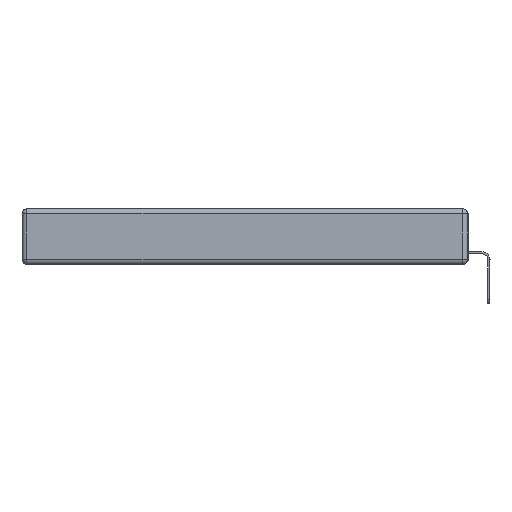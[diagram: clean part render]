
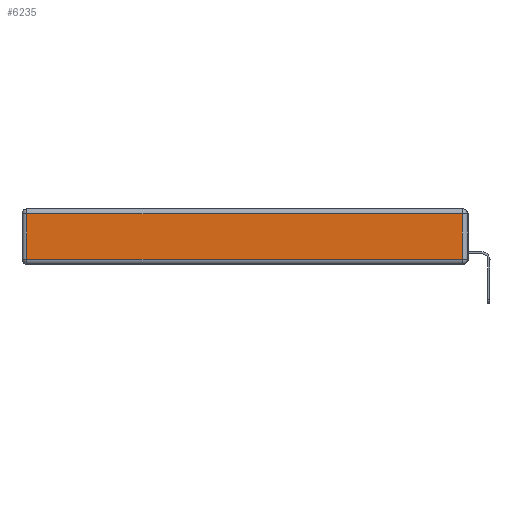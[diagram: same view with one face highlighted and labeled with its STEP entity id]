
A CAD part, left-side view. The second image highlights one B-rep face of the part: STEP entity #6235.
In plain terms, the highlighted planar face has unit normal (-1, 0, 0).
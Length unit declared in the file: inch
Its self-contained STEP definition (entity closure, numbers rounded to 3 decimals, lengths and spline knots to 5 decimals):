
#441 = VECTOR ( 'NONE', #6991, 39.37008 ) ;
#1010 = AXIS2_PLACEMENT_3D ( 'NONE', #11171, #18867, #4744 ) ;
#1175 = FACE_OUTER_BOUND ( 'NONE', #8351, .T. ) ;
#1497 = VERTEX_POINT ( 'NONE', #19045 ) ;
#2666 = DIRECTION ( 'NONE',  ( 0., 0., -1. ) ) ;
#3133 = PLANE ( 'NONE',  #1010 ) ;
#4744 = DIRECTION ( 'NONE',  ( 0., 0., 1. ) ) ;
#5051 = VERTEX_POINT ( 'NONE', #17936 ) ;
#5060 = DIRECTION ( 'NONE',  ( 0., -1., 0. ) ) ;
#5357 = VECTOR ( 'NONE', #15105, 39.37008 ) ;
#5950 = CARTESIAN_POINT ( 'NONE',  ( 0., 2.72, -0.343 ) ) ;
#6235 = ADVANCED_FACE ( 'NONE', ( #1175 ), #3133, .T. ) ;
#6850 = EDGE_CURVE ( 'NONE', #5051, #15081, #16996, .T. ) ;
#6991 = DIRECTION ( 'NONE',  ( 0., 1., 0. ) ) ;
#8351 = EDGE_LOOP ( 'NONE', ( #13451, #8985, #16071, #19048 ) ) ;
#8985 = ORIENTED_EDGE ( 'NONE', *, *, #14869, .T. ) ;
#9962 = CARTESIAN_POINT ( 'NONE',  ( 0., 0.03, -0.03 ) ) ;
#10118 = LINE ( 'NONE', #14499, #5357 ) ;
#11171 = CARTESIAN_POINT ( 'NONE',  ( 0., 0., -0.343 ) ) ;
#12947 = EDGE_CURVE ( 'NONE', #17472, #1497, #17283, .T. ) ;
#13451 = ORIENTED_EDGE ( 'NONE', *, *, #6850, .T. ) ;
#14499 = CARTESIAN_POINT ( 'NONE',  ( 0., 0.03, -0.343 ) ) ;
#14869 = EDGE_CURVE ( 'NONE', #15081, #17472, #10118, .T. ) ;
#15017 = VECTOR ( 'NONE', #5060, 39.37008 ) ;
#15081 = VERTEX_POINT ( 'NONE', #15450 ) ;
#15105 = DIRECTION ( 'NONE',  ( 0., 0., 1. ) ) ;
#15450 = CARTESIAN_POINT ( 'NONE',  ( 0., 0.03, -0.313 ) ) ;
#15905 = VECTOR ( 'NONE', #2666, 39.37008 ) ;
#16071 = ORIENTED_EDGE ( 'NONE', *, *, #12947, .T. ) ;
#16996 = LINE ( 'NONE', #17722, #15017 ) ;
#17283 = LINE ( 'NONE', #19730, #441 ) ;
#17472 = VERTEX_POINT ( 'NONE', #9962 ) ;
#17710 = EDGE_CURVE ( 'NONE', #1497, #5051, #18639, .T. ) ;
#17722 = CARTESIAN_POINT ( 'NONE',  ( 0., 0., -0.313 ) ) ;
#17936 = CARTESIAN_POINT ( 'NONE',  ( 0., 2.72, -0.313 ) ) ;
#18639 = LINE ( 'NONE', #5950, #15905 ) ;
#18867 = DIRECTION ( 'NONE',  ( -1., 0., 0. ) ) ;
#19045 = CARTESIAN_POINT ( 'NONE',  ( 0., 2.72, -0.03 ) ) ;
#19048 = ORIENTED_EDGE ( 'NONE', *, *, #17710, .T. ) ;
#19730 = CARTESIAN_POINT ( 'NONE',  ( 0., 2.75, -0.03 ) ) ;
